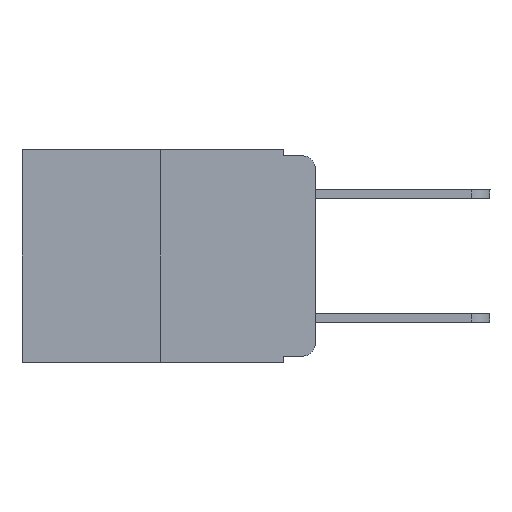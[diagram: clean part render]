
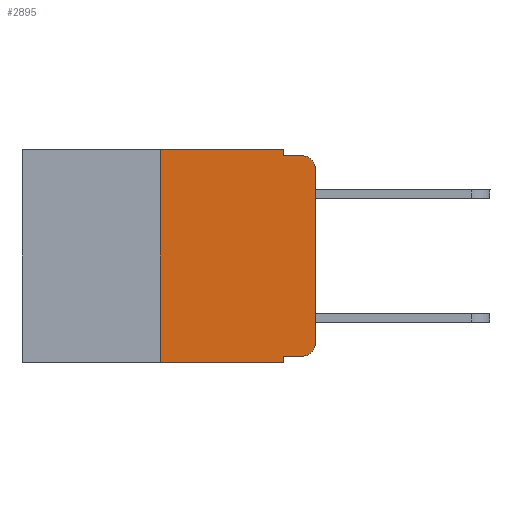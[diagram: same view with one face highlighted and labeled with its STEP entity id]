
A CAD part, left-side view. The second image highlights one B-rep face of the part: STEP entity #2895.
In plain terms, the highlighted planar face has unit normal (-1, 0, 0).
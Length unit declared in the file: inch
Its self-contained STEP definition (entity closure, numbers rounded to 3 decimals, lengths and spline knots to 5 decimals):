
#14 = EDGE_LOOP ( 'NONE', ( #4464, #5453, #4171, #9100, #9344, #13272, #1925, #14259, #2162, #1726 ) ) ;
#264 = CARTESIAN_POINT ( 'NONE',  ( 0., 0.051, 0. ) ) ;
#521 = VECTOR ( 'NONE', #2913, 39.37008 ) ;
#556 = LINE ( 'NONE', #13328, #12953 ) ;
#1001 = AXIS2_PLACEMENT_3D ( 'NONE', #14434, #11058, #7443 ) ;
#1176 = CARTESIAN_POINT ( 'NONE',  ( 0., 0.02, -0.03 ) ) ;
#1444 = CARTESIAN_POINT ( 'NONE',  ( 0., 0.051, -0.343 ) ) ;
#1574 = EDGE_CURVE ( 'NONE', #5787, #14698, #3776, .T. ) ;
#1647 = VECTOR ( 'NONE', #7054, 39.37008 ) ;
#1726 = ORIENTED_EDGE ( 'NONE', *, *, #14300, .T. ) ;
#1925 = ORIENTED_EDGE ( 'NONE', *, *, #6120, .T. ) ;
#2162 = ORIENTED_EDGE ( 'NONE', *, *, #14706, .T. ) ;
#2403 = VERTEX_POINT ( 'NONE', #1444 ) ;
#2651 = CARTESIAN_POINT ( 'NONE',  ( 0., 0.473, 0. ) ) ;
#2685 = VECTOR ( 'NONE', #10555, 39.37008 ) ;
#2698 = LINE ( 'NONE', #7424, #521 ) ;
#2895 = ADVANCED_FACE ( 'NONE', ( #5149 ), #9844, .F. ) ;
#2913 = DIRECTION ( 'NONE',  ( 0., -1., 0. ) ) ;
#3089 = DIRECTION ( 'NONE',  ( 0., -1., 0. ) ) ;
#3212 = CARTESIAN_POINT ( 'NONE',  ( 0., 0., -0.313 ) ) ;
#3328 = VECTOR ( 'NONE', #11235, 39.37008 ) ;
#3414 = CARTESIAN_POINT ( 'NONE',  ( 0., 0.25, 0. ) ) ;
#3644 = LINE ( 'NONE', #3723, #2685 ) ;
#3723 = CARTESIAN_POINT ( 'NONE',  ( 0., 0.051, -0.01 ) ) ;
#3776 = LINE ( 'NONE', #14445, #7284 ) ;
#3823 = VECTOR ( 'NONE', #8662, 39.37008 ) ;
#3854 = DIRECTION ( 'NONE',  ( 0., 0., -1. ) ) ;
#4171 = ORIENTED_EDGE ( 'NONE', *, *, #11610, .F. ) ;
#4464 = ORIENTED_EDGE ( 'NONE', *, *, #7383, .T. ) ;
#4575 = VERTEX_POINT ( 'NONE', #10605 ) ;
#4748 = VERTEX_POINT ( 'NONE', #6426 ) ;
#4820 = CIRCLE ( 'NONE', #13397, 0.02 ) ;
#5059 = VERTEX_POINT ( 'NONE', #12726 ) ;
#5149 = FACE_OUTER_BOUND ( 'NONE', #14, .T. ) ;
#5208 = LINE ( 'NONE', #14574, #3823 ) ;
#5453 = ORIENTED_EDGE ( 'NONE', *, *, #10627, .T. ) ;
#5787 = VERTEX_POINT ( 'NONE', #3414 ) ;
#5799 = DIRECTION ( 'NONE',  ( 0., 0., -1. ) ) ;
#6094 = VERTEX_POINT ( 'NONE', #14377 ) ;
#6120 = EDGE_CURVE ( 'NONE', #5059, #2403, #10061, .T. ) ;
#6426 = CARTESIAN_POINT ( 'NONE',  ( 0., 0.02, -0.01 ) ) ;
#7054 = DIRECTION ( 'NONE',  ( 0., 0., -1. ) ) ;
#7284 = VECTOR ( 'NONE', #10847, 39.37008 ) ;
#7383 = EDGE_CURVE ( 'NONE', #9698, #10538, #9931, .T. ) ;
#7424 = CARTESIAN_POINT ( 'NONE',  ( 0., 0.051, -0.333 ) ) ;
#7443 = DIRECTION ( 'NONE',  ( 0., 0., -1. ) ) ;
#7496 = DIRECTION ( 'NONE',  ( 0., 0., 1. ) ) ;
#7577 = CARTESIAN_POINT ( 'NONE',  ( 0., 0.051, 0. ) ) ;
#7666 = EDGE_CURVE ( 'NONE', #14698, #7730, #5208, .T. ) ;
#7730 = VERTEX_POINT ( 'NONE', #11995 ) ;
#8199 = DIRECTION ( 'NONE',  ( -1., 0., 0. ) ) ;
#8662 = DIRECTION ( 'NONE',  ( 0., 0., -1. ) ) ;
#9100 = ORIENTED_EDGE ( 'NONE', *, *, #7666, .F. ) ;
#9344 = ORIENTED_EDGE ( 'NONE', *, *, #1574, .F. ) ;
#9462 = EDGE_CURVE ( 'NONE', #4575, #2403, #10739, .T. ) ;
#9698 = VERTEX_POINT ( 'NONE', #3212 ) ;
#9844 = PLANE ( 'NONE',  #13234 ) ;
#9931 = LINE ( 'NONE', #14469, #3328 ) ;
#10061 = LINE ( 'NONE', #13514, #14055 ) ;
#10538 = VERTEX_POINT ( 'NONE', #12364 ) ;
#10555 = DIRECTION ( 'NONE',  ( 0., -1., 0. ) ) ;
#10605 = CARTESIAN_POINT ( 'NONE',  ( 0., 0.051, -0.333 ) ) ;
#10627 = EDGE_CURVE ( 'NONE', #10538, #4748, #4820, .T. ) ;
#10739 = LINE ( 'NONE', #264, #1647 ) ;
#10847 = DIRECTION ( 'NONE',  ( 0., -1., 0. ) ) ;
#11026 = CIRCLE ( 'NONE', #1001, 0.02 ) ;
#11058 = DIRECTION ( 'NONE',  ( -1., 0., 0. ) ) ;
#11235 = DIRECTION ( 'NONE',  ( 0., 0., 1. ) ) ;
#11610 = EDGE_CURVE ( 'NONE', #7730, #4748, #3644, .T. ) ;
#11995 = CARTESIAN_POINT ( 'NONE',  ( 0., 0.051, -0.01 ) ) ;
#12364 = CARTESIAN_POINT ( 'NONE',  ( 0., 0., -0.03 ) ) ;
#12726 = CARTESIAN_POINT ( 'NONE',  ( 0., 0.25, -0.343 ) ) ;
#12953 = VECTOR ( 'NONE', #7496, 39.37008 ) ;
#13234 = AXIS2_PLACEMENT_3D ( 'NONE', #2651, #14518, #3854 ) ;
#13272 = ORIENTED_EDGE ( 'NONE', *, *, #13494, .F. ) ;
#13328 = CARTESIAN_POINT ( 'NONE',  ( 0., 0.25, 0. ) ) ;
#13397 = AXIS2_PLACEMENT_3D ( 'NONE', #1176, #8199, #5799 ) ;
#13494 = EDGE_CURVE ( 'NONE', #5059, #5787, #556, .T. ) ;
#13514 = CARTESIAN_POINT ( 'NONE',  ( 0., 0.473, -0.343 ) ) ;
#14055 = VECTOR ( 'NONE', #3089, 39.37008 ) ;
#14259 = ORIENTED_EDGE ( 'NONE', *, *, #9462, .F. ) ;
#14300 = EDGE_CURVE ( 'NONE', #6094, #9698, #11026, .T. ) ;
#14377 = CARTESIAN_POINT ( 'NONE',  ( 0., 0.02, -0.333 ) ) ;
#14434 = CARTESIAN_POINT ( 'NONE',  ( 0., 0.02, -0.313 ) ) ;
#14445 = CARTESIAN_POINT ( 'NONE',  ( 0., 0.473, 0. ) ) ;
#14469 = CARTESIAN_POINT ( 'NONE',  ( 0., 0., 0. ) ) ;
#14518 = DIRECTION ( 'NONE',  ( 1., 0., 0. ) ) ;
#14574 = CARTESIAN_POINT ( 'NONE',  ( 0., 0.051, 0. ) ) ;
#14698 = VERTEX_POINT ( 'NONE', #7577 ) ;
#14706 = EDGE_CURVE ( 'NONE', #4575, #6094, #2698, .T. ) ;
